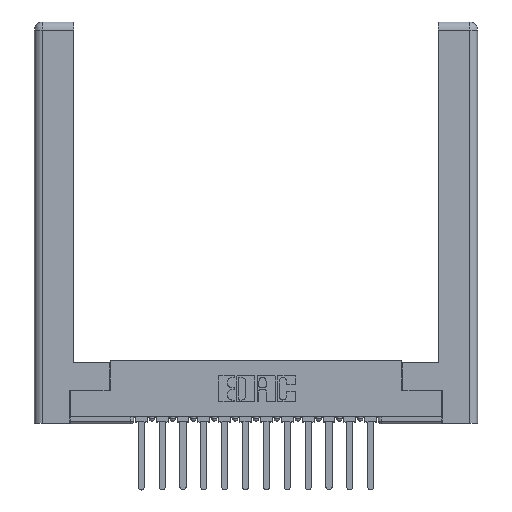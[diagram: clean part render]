
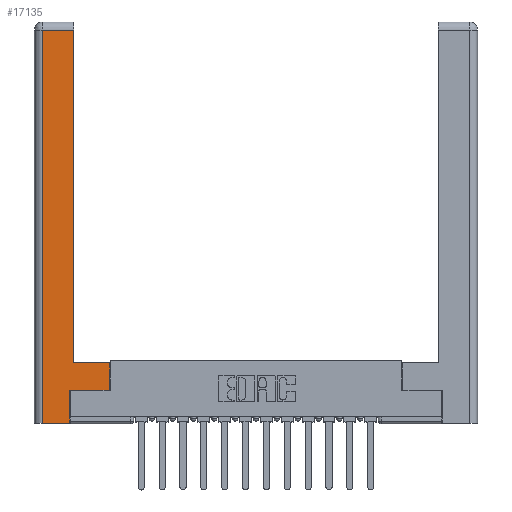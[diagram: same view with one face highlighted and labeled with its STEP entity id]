
A CAD part, top view. The second image highlights one B-rep face of the part: STEP entity #17135.
In plain terms, the highlighted planar face has unit normal (0, 0, 1).
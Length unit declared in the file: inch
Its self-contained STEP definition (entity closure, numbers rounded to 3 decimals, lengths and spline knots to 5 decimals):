
#217 = CARTESIAN_POINT ( 'NONE',  ( 0.295, 3., 0. ) ) ;
#622 = ORIENTED_EDGE ( 'NONE', *, *, #16347, .T. ) ;
#822 = VERTEX_POINT ( 'NONE', #2874 ) ;
#1322 = ORIENTED_EDGE ( 'NONE', *, *, #6868, .T. ) ;
#1344 = VECTOR ( 'NONE', #2360, 39.37008 ) ;
#1598 = CARTESIAN_POINT ( 'NONE',  ( 0.265, 0.245, 0. ) ) ;
#1653 = DIRECTION ( 'NONE',  ( 0., 1., 0. ) ) ;
#1773 = DIRECTION ( 'NONE',  ( 1., 0., 0. ) ) ;
#2360 = DIRECTION ( 'NONE',  ( 0., 1., 0. ) ) ;
#2870 = VECTOR ( 'NONE', #1653, 39.37008 ) ;
#2874 = CARTESIAN_POINT ( 'NONE',  ( 0.295, 0.45, 0. ) ) ;
#2996 = LINE ( 'NONE', #13765, #4888 ) ;
#3701 = LINE ( 'NONE', #217, #4955 ) ;
#3990 = DIRECTION ( 'NONE',  ( 0., 0., -1. ) ) ;
#4041 = CARTESIAN_POINT ( 'NONE',  ( 0.0615, 0., 0. ) ) ;
#4112 = PLANE ( 'NONE',  #5600 ) ;
#4419 = EDGE_CURVE ( 'NONE', #822, #7765, #3701, .T. ) ;
#4488 = CARTESIAN_POINT ( 'NONE',  ( 0.565, 0.45, 0. ) ) ;
#4726 = VERTEX_POINT ( 'NONE', #15403 ) ;
#4888 = VECTOR ( 'NONE', #1773, 39.37008 ) ;
#4955 = VECTOR ( 'NONE', #10845, 39.37008 ) ;
#5166 = CARTESIAN_POINT ( 'NONE',  ( 0.0615, 0., 0. ) ) ;
#5225 = VERTEX_POINT ( 'NONE', #5166 ) ;
#5336 = DIRECTION ( 'NONE',  ( -1., 0., 0. ) ) ;
#5517 = VERTEX_POINT ( 'NONE', #10033 ) ;
#5600 = AXIS2_PLACEMENT_3D ( 'NONE', #12200, #3990, #5336 ) ;
#5911 = ORIENTED_EDGE ( 'NONE', *, *, #10727, .T. ) ;
#6350 = CARTESIAN_POINT ( 'NONE',  ( 0.295, 2.94, 0. ) ) ;
#6399 = CARTESIAN_POINT ( 'NONE',  ( 0.565, 0.45, 0. ) ) ;
#6435 = ORIENTED_EDGE ( 'NONE', *, *, #12679, .T. ) ;
#6448 = VECTOR ( 'NONE', #11478, 39.37008 ) ;
#6550 = VERTEX_POINT ( 'NONE', #17064 ) ;
#6565 = ORIENTED_EDGE ( 'NONE', *, *, #4419, .T. ) ;
#6868 = EDGE_CURVE ( 'NONE', #6550, #4726, #2996, .T. ) ;
#7215 = EDGE_CURVE ( 'NONE', #8278, #5225, #15306, .T. ) ;
#7352 = ORIENTED_EDGE ( 'NONE', *, *, #16779, .T. ) ;
#7765 = VERTEX_POINT ( 'NONE', #6350 ) ;
#8278 = VERTEX_POINT ( 'NONE', #9038 ) ;
#8792 = DIRECTION ( 'NONE',  ( 1., 0., 0. ) ) ;
#9038 = CARTESIAN_POINT ( 'NONE',  ( 0.0615, 2.94, 0. ) ) ;
#9125 = ORIENTED_EDGE ( 'NONE', *, *, #7215, .T. ) ;
#9604 = EDGE_CURVE ( 'NONE', #7765, #8278, #16492, .T. ) ;
#10033 = CARTESIAN_POINT ( 'NONE',  ( 0.265, 0., 0. ) ) ;
#10727 = EDGE_CURVE ( 'NONE', #5517, #6550, #13930, .T. ) ;
#10845 = DIRECTION ( 'NONE',  ( 0., 1., 0. ) ) ;
#11298 = VERTEX_POINT ( 'NONE', #4488 ) ;
#11478 = DIRECTION ( 'NONE',  ( -1., 0., 0. ) ) ;
#11580 = FACE_OUTER_BOUND ( 'NONE', #11735, .T. ) ;
#11637 = CARTESIAN_POINT ( 'NONE',  ( 0.265, 0., 0. ) ) ;
#11735 = EDGE_LOOP ( 'NONE', ( #6565, #13033, #9125, #7352, #5911, #1322, #6435, #622 ) ) ;
#12200 = CARTESIAN_POINT ( 'NONE',  ( 0., 0., 0. ) ) ;
#12311 = DIRECTION ( 'NONE',  ( -1., 0., 0. ) ) ;
#12371 = VECTOR ( 'NONE', #14638, 39.37008 ) ;
#12679 = EDGE_CURVE ( 'NONE', #4726, #11298, #16851, .T. ) ;
#13033 = ORIENTED_EDGE ( 'NONE', *, *, #9604, .T. ) ;
#13765 = CARTESIAN_POINT ( 'NONE',  ( 0.565, 0.245, 0. ) ) ;
#13930 = LINE ( 'NONE', #1598, #2870 ) ;
#14159 = VECTOR ( 'NONE', #12311, 39.37008 ) ;
#14294 = VECTOR ( 'NONE', #8792, 39.37008 ) ;
#14638 = DIRECTION ( 'NONE',  ( 0., -1., 0. ) ) ;
#15176 = CARTESIAN_POINT ( 'NONE',  ( 0.0615, 2.94, 0. ) ) ;
#15306 = LINE ( 'NONE', #4041, #12371 ) ;
#15345 = LINE ( 'NONE', #11637, #14294 ) ;
#15403 = CARTESIAN_POINT ( 'NONE',  ( 0.565, 0.245, 0. ) ) ;
#16347 = EDGE_CURVE ( 'NONE', #11298, #822, #17154, .T. ) ;
#16492 = LINE ( 'NONE', #15176, #14159 ) ;
#16762 = CARTESIAN_POINT ( 'NONE',  ( 0.295, 0.45, 0. ) ) ;
#16779 = EDGE_CURVE ( 'NONE', #5225, #5517, #15345, .T. ) ;
#16851 = LINE ( 'NONE', #6399, #1344 ) ;
#17064 = CARTESIAN_POINT ( 'NONE',  ( 0.265, 0.245, 0. ) ) ;
#17135 = ADVANCED_FACE ( 'NONE', ( #11580 ), #4112, .F. ) ;
#17154 = LINE ( 'NONE', #16762, #6448 ) ;
